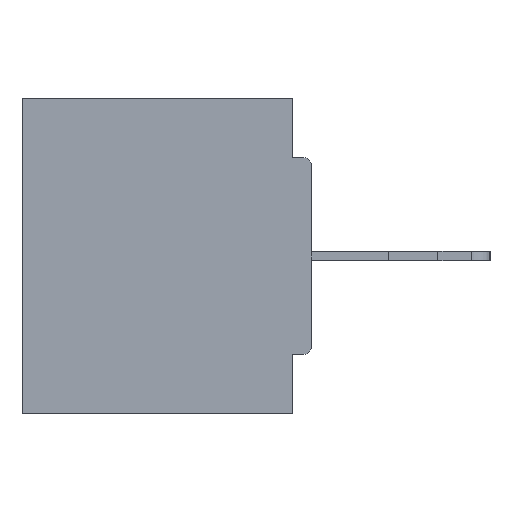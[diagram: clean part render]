
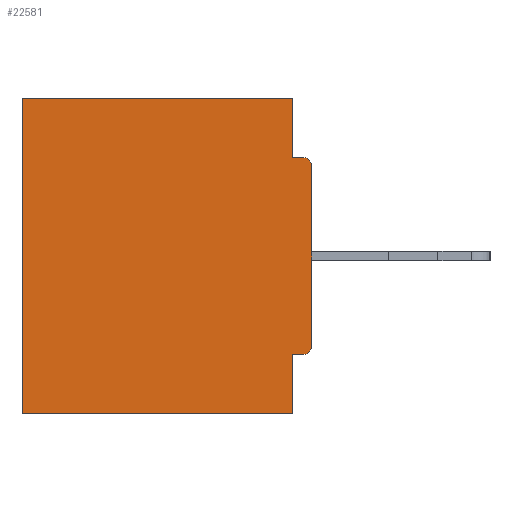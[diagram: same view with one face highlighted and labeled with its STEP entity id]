
A CAD part, left-side view. The second image highlights one B-rep face of the part: STEP entity #22581.
In plain terms, the highlighted planar face has unit normal (-1, 0, 0).
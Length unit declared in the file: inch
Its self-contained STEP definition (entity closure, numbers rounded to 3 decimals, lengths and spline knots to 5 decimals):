
#18 = VECTOR ( 'NONE', #10703, 39.37008 ) ;
#154 = DIRECTION ( 'NONE',  ( 0., 0., -1. ) ) ;
#204 = VERTEX_POINT ( 'NONE', #20276 ) ;
#800 = ORIENTED_EDGE ( 'NONE', *, *, #26074, .F. ) ;
#941 = ORIENTED_EDGE ( 'NONE', *, *, #2887, .F. ) ;
#1846 = VERTEX_POINT ( 'NONE', #8204 ) ;
#1960 = ORIENTED_EDGE ( 'NONE', *, *, #7295, .T. ) ;
#2374 = LINE ( 'NONE', #25741, #21031 ) ;
#2686 = CIRCLE ( 'NONE', #5386, 0.015 ) ;
#2776 = ORIENTED_EDGE ( 'NONE', *, *, #8723, .T. ) ;
#2811 = CARTESIAN_POINT ( 'NONE',  ( 0.298, 0., 0. ) ) ;
#2843 = CARTESIAN_POINT ( 'NONE',  ( 0.298, 0., -0.4065 ) ) ;
#2887 = EDGE_CURVE ( 'NONE', #5998, #11000, #7308, .T. ) ;
#3277 = EDGE_CURVE ( 'NONE', #3686, #5387, #8383, .T. ) ;
#3484 = PLANE ( 'NONE',  #15532 ) ;
#3529 = VECTOR ( 'NONE', #12626, 39.37008 ) ;
#3686 = VERTEX_POINT ( 'NONE', #6708 ) ;
#3789 = VERTEX_POINT ( 'NONE', #26522 ) ;
#4034 = ORIENTED_EDGE ( 'NONE', *, *, #29781, .F. ) ;
#4955 = VERTEX_POINT ( 'NONE', #18721 ) ;
#5386 = AXIS2_PLACEMENT_3D ( 'NONE', #30914, #16738, #154 ) ;
#5387 = VERTEX_POINT ( 'NONE', #20262 ) ;
#5442 = CARTESIAN_POINT ( 'NONE',  ( 0.298, 0.031, -0.0935 ) ) ;
#5831 = CARTESIAN_POINT ( 'NONE',  ( 0.298, 0.46, 0. ) ) ;
#5900 = DIRECTION ( 'NONE',  ( 0., 0., -1. ) ) ;
#5949 = VECTOR ( 'NONE', #7687, 39.37008 ) ;
#5998 = VERTEX_POINT ( 'NONE', #5442 ) ;
#6321 = DIRECTION ( 'NONE',  ( 0., 1., 0. ) ) ;
#6708 = CARTESIAN_POINT ( 'NONE',  ( 0.298, 0.015, -0.4065 ) ) ;
#7169 = CARTESIAN_POINT ( 'NONE',  ( 0.298, 0., -0.0935 ) ) ;
#7295 = EDGE_CURVE ( 'NONE', #13161, #11000, #21625, .T. ) ;
#7308 = LINE ( 'NONE', #7169, #25639 ) ;
#7687 = DIRECTION ( 'NONE',  ( 0., 0., -1. ) ) ;
#8181 = LINE ( 'NONE', #2811, #5949 ) ;
#8204 = CARTESIAN_POINT ( 'NONE',  ( 0.298, 0., -0.3915 ) ) ;
#8383 = LINE ( 'NONE', #2843, #3529 ) ;
#8387 = DIRECTION ( 'NONE',  ( 1., 0., 0. ) ) ;
#8723 = EDGE_CURVE ( 'NONE', #4955, #3789, #18239, .T. ) ;
#10703 = DIRECTION ( 'NONE',  ( 0., 0., -1. ) ) ;
#11000 = VERTEX_POINT ( 'NONE', #14523 ) ;
#11712 = FACE_OUTER_BOUND ( 'NONE', #17278, .T. ) ;
#11858 = CARTESIAN_POINT ( 'NONE',  ( 0.298, 0.031, -0.5 ) ) ;
#12626 = DIRECTION ( 'NONE',  ( 0., 1., 0. ) ) ;
#12745 = CARTESIAN_POINT ( 'NONE',  ( 0.298, 0.031, -0.5 ) ) ;
#13161 = VERTEX_POINT ( 'NONE', #30181 ) ;
#13760 = LINE ( 'NONE', #29589, #21623 ) ;
#14523 = CARTESIAN_POINT ( 'NONE',  ( 0.298, 0.015, -0.0935 ) ) ;
#15532 = AXIS2_PLACEMENT_3D ( 'NONE', #22794, #8387, #5900 ) ;
#15823 = EDGE_CURVE ( 'NONE', #13161, #1846, #8181, .T. ) ;
#16034 = ORIENTED_EDGE ( 'NONE', *, *, #16588, .F. ) ;
#16588 = EDGE_CURVE ( 'NONE', #26692, #204, #13760, .T. ) ;
#16738 = DIRECTION ( 'NONE',  ( -1., 0., 0. ) ) ;
#17278 = EDGE_LOOP ( 'NONE', ( #1960, #941, #800, #2776, #22808, #16034, #4034, #19529, #22538, #17923 ) ) ;
#17632 = DIRECTION ( 'NONE',  ( 0., 1., 0. ) ) ;
#17923 = ORIENTED_EDGE ( 'NONE', *, *, #15823, .F. ) ;
#18065 = CARTESIAN_POINT ( 'NONE',  ( 0.298, 0., 0. ) ) ;
#18156 = DIRECTION ( 'NONE',  ( 0., 0., -1. ) ) ;
#18239 = LINE ( 'NONE', #18065, #20884 ) ;
#18508 = DIRECTION ( 'NONE',  ( 0., 0., -1. ) ) ;
#18721 = CARTESIAN_POINT ( 'NONE',  ( 0.298, 0.031, 0. ) ) ;
#19529 = ORIENTED_EDGE ( 'NONE', *, *, #3277, .F. ) ;
#20262 = CARTESIAN_POINT ( 'NONE',  ( 0.298, 0.031, -0.4065 ) ) ;
#20276 = CARTESIAN_POINT ( 'NONE',  ( 0.298, 0.46, -0.5 ) ) ;
#20669 = AXIS2_PLACEMENT_3D ( 'NONE', #28605, #25571, #18508 ) ;
#20884 = VECTOR ( 'NONE', #6321, 39.37008 ) ;
#21031 = VECTOR ( 'NONE', #18156, 39.37008 ) ;
#21623 = VECTOR ( 'NONE', #17632, 39.37008 ) ;
#21625 = CIRCLE ( 'NONE', #20669, 0.015 ) ;
#22428 = LINE ( 'NONE', #11858, #31038 ) ;
#22538 = ORIENTED_EDGE ( 'NONE', *, *, #29759, .T. ) ;
#22581 = ADVANCED_FACE ( 'NONE', ( #11712 ), #3484, .F. ) ;
#22794 = CARTESIAN_POINT ( 'NONE',  ( 0.298, 0., 0. ) ) ;
#22808 = ORIENTED_EDGE ( 'NONE', *, *, #27148, .T. ) ;
#25571 = DIRECTION ( 'NONE',  ( -1., 0., 0. ) ) ;
#25639 = VECTOR ( 'NONE', #28677, 39.37008 ) ;
#25741 = CARTESIAN_POINT ( 'NONE',  ( 0.298, 0.031, -0.5 ) ) ;
#26074 = EDGE_CURVE ( 'NONE', #4955, #5998, #2374, .T. ) ;
#26517 = DIRECTION ( 'NONE',  ( 0., 0., -1. ) ) ;
#26522 = CARTESIAN_POINT ( 'NONE',  ( 0.298, 0.46, 0. ) ) ;
#26692 = VERTEX_POINT ( 'NONE', #12745 ) ;
#27148 = EDGE_CURVE ( 'NONE', #3789, #204, #28459, .T. ) ;
#28459 = LINE ( 'NONE', #5831, #18 ) ;
#28605 = CARTESIAN_POINT ( 'NONE',  ( 0.298, 0.015, -0.1085 ) ) ;
#28677 = DIRECTION ( 'NONE',  ( 0., -1., 0. ) ) ;
#29589 = CARTESIAN_POINT ( 'NONE',  ( 0.298, 0., -0.5 ) ) ;
#29759 = EDGE_CURVE ( 'NONE', #3686, #1846, #2686, .T. ) ;
#29781 = EDGE_CURVE ( 'NONE', #5387, #26692, #22428, .T. ) ;
#30181 = CARTESIAN_POINT ( 'NONE',  ( 0.298, 0., -0.1085 ) ) ;
#30914 = CARTESIAN_POINT ( 'NONE',  ( 0.298, 0.015, -0.3915 ) ) ;
#31038 = VECTOR ( 'NONE', #26517, 39.37008 ) ;
